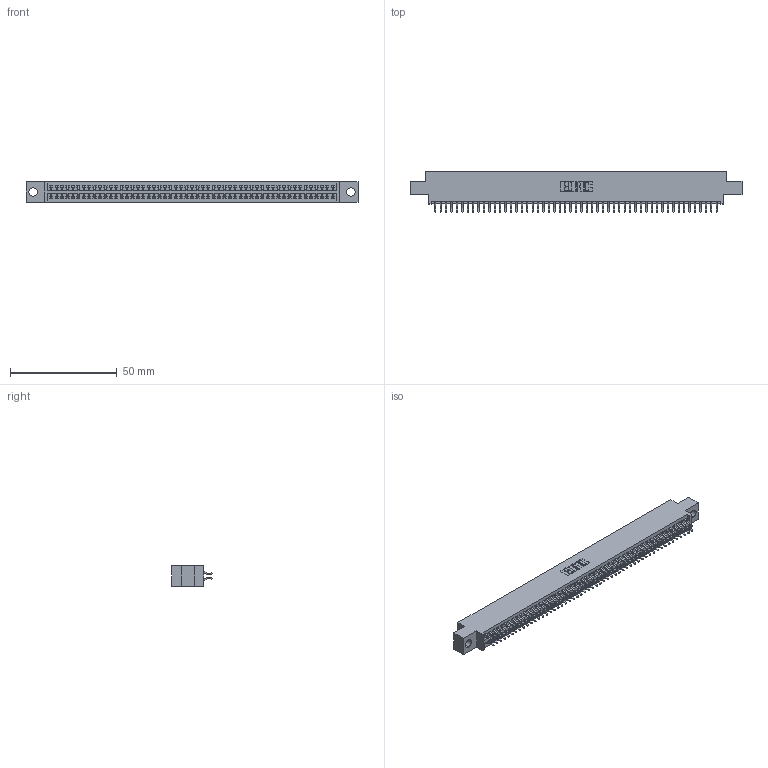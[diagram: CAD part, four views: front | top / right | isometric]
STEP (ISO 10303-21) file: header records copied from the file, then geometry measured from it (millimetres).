
FILE_DESCRIPTION (( 'STEP AP203' ), '1' );
FILE_NAME ('345-106-556-804.STEP', '2018-10-07T03:43:46', ( '' ), ( '' ), 'SwSTEP 2.0', 'SolidWorks 2016', '' );
FILE_SCHEMA (( 'CONFIG_CONTROL_DESIGN' ));
Length unit declared in the file: inch
Products named in the file (3): 345 Part_0.170 Offset - 0.156 Dia-TH; 345-292-001_556 Tail; 345-106-556-804
Assembly tree (107 placements, depth 2):
  345-106-556-804
    345 Part_0.170 Offset - 0.156 Dia-TH
    345-292-001_556 Tail  x106
Bounding box: 155.83 x 19.24 x 9.4 mm (x, y, z)
Volume: 15034.1 mm3; surface area: 22301.8 mm2
Topology: 107 solids, 107 shells, 6066 faces, 18055 edges, 11894 vertices
Faces by surface type: plane 4006, cylinder 2060
Entity records: 40459 total; most frequent: CARTESIAN_POINT 6788, ORIENTED_EDGE 6710, DIRECTION 5959, EDGE_CURVE 3355, VECTOR 3003, LINE 3003, VERTEX_POINT 2234, AXIS2_PLACEMENT_3D 1478
